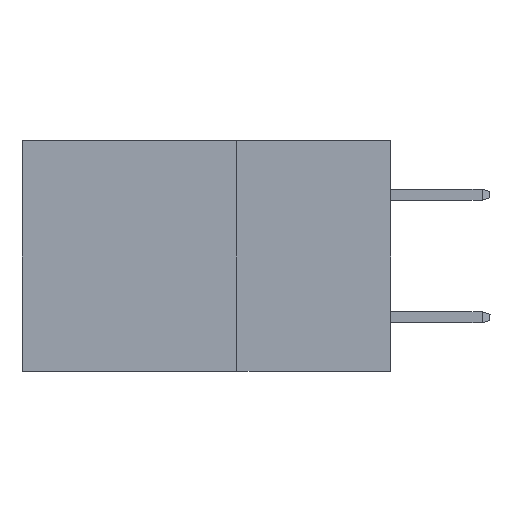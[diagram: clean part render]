
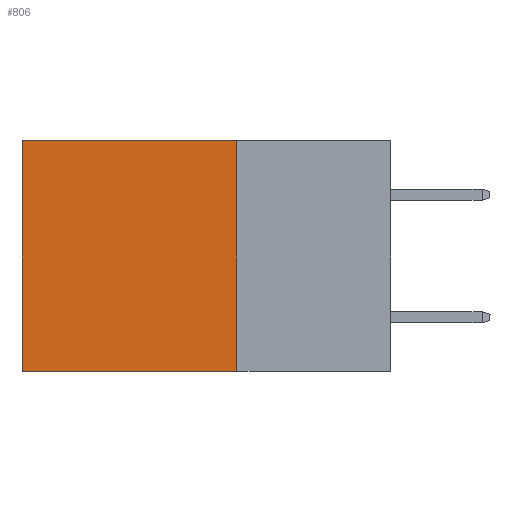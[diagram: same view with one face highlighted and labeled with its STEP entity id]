
A CAD part, left-side view. The second image highlights one B-rep face of the part: STEP entity #806.
In plain terms, the highlighted planar face has unit normal (-1, 0, 0).
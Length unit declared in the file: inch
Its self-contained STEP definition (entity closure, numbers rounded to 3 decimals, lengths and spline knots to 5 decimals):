
#792 = ORIENTED_EDGE ( 'NONE', *, *, #11207, .F. ) ;
#806 = ADVANCED_FACE ( 'NONE', ( #13488 ), #1959, .F. ) ;
#1088 = EDGE_LOOP ( 'NONE', ( #16945, #9734, #792, #12178 ) ) ;
#1959 = PLANE ( 'NONE',  #16507 ) ;
#1979 = VECTOR ( 'NONE', #13370, 39.37008 ) ;
#2175 = CARTESIAN_POINT ( 'NONE',  ( 0.2875, 0.6, -0.375 ) ) ;
#3043 = CARTESIAN_POINT ( 'NONE',  ( 0.2875, 0.25, -0.375 ) ) ;
#3511 = VERTEX_POINT ( 'NONE', #16765 ) ;
#3841 = VECTOR ( 'NONE', #12674, 39.37008 ) ;
#4036 = LINE ( 'NONE', #3043, #1979 ) ;
#4414 = CARTESIAN_POINT ( 'NONE',  ( 0.2875, 0.25, -0.375 ) ) ;
#4557 = LINE ( 'NONE', #6193, #6782 ) ;
#5243 = CARTESIAN_POINT ( 'NONE',  ( 0.2875, 0.25, 0. ) ) ;
#5917 = DIRECTION ( 'NONE',  ( 1., 0., 0. ) ) ;
#6193 = CARTESIAN_POINT ( 'NONE',  ( 0.2875, 0.25, 0. ) ) ;
#6257 = LINE ( 'NONE', #15535, #9739 ) ;
#6782 = VECTOR ( 'NONE', #15372, 39.37008 ) ;
#7109 = LINE ( 'NONE', #2175, #3841 ) ;
#8119 = VERTEX_POINT ( 'NONE', #4414 ) ;
#8335 = CARTESIAN_POINT ( 'NONE',  ( 0.2875, 0.25, -0.375 ) ) ;
#9734 = ORIENTED_EDGE ( 'NONE', *, *, #10979, .F. ) ;
#9739 = VECTOR ( 'NONE', #15468, 39.37008 ) ;
#10613 = EDGE_CURVE ( 'NONE', #13130, #3511, #7109, .T. ) ;
#10979 = EDGE_CURVE ( 'NONE', #8119, #3511, #4036, .T. ) ;
#11129 = DIRECTION ( 'NONE',  ( 0., 0., -1. ) ) ;
#11207 = EDGE_CURVE ( 'NONE', #16660, #8119, #6257, .T. ) ;
#12178 = ORIENTED_EDGE ( 'NONE', *, *, #14339, .T. ) ;
#12674 = DIRECTION ( 'NONE',  ( 0., 0., -1. ) ) ;
#13130 = VERTEX_POINT ( 'NONE', #13877 ) ;
#13370 = DIRECTION ( 'NONE',  ( 0., 1., 0. ) ) ;
#13488 = FACE_OUTER_BOUND ( 'NONE', #1088, .T. ) ;
#13877 = CARTESIAN_POINT ( 'NONE',  ( 0.2875, 0.6, 0. ) ) ;
#14339 = EDGE_CURVE ( 'NONE', #16660, #13130, #4557, .T. ) ;
#15372 = DIRECTION ( 'NONE',  ( 0., 1., 0. ) ) ;
#15468 = DIRECTION ( 'NONE',  ( 0., 0., -1. ) ) ;
#15535 = CARTESIAN_POINT ( 'NONE',  ( 0.2875, 0.25, -0.375 ) ) ;
#16507 = AXIS2_PLACEMENT_3D ( 'NONE', #8335, #5917, #11129 ) ;
#16660 = VERTEX_POINT ( 'NONE', #5243 ) ;
#16765 = CARTESIAN_POINT ( 'NONE',  ( 0.2875, 0.6, -0.375 ) ) ;
#16945 = ORIENTED_EDGE ( 'NONE', *, *, #10613, .T. ) ;
